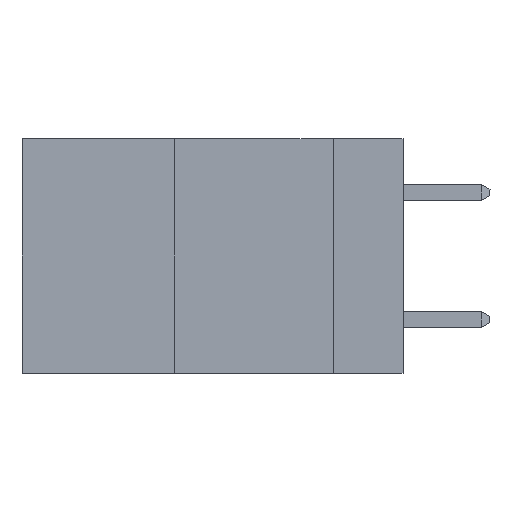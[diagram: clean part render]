
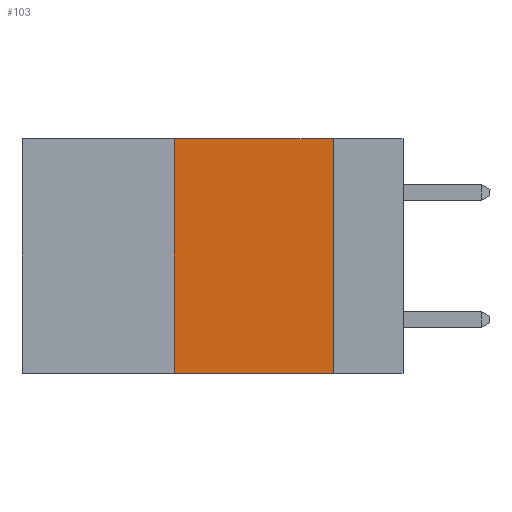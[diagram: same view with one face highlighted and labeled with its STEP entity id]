
A CAD part, left-side view. The second image highlights one B-rep face of the part: STEP entity #103.
In plain terms, the highlighted planar face has unit normal (-1, 0, 0).
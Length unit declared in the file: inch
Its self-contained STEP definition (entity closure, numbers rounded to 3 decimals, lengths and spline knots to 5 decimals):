
#28 = LINE ( 'NONE', #5893, #8463 ) ;
#103 = ADVANCED_FACE ( 'NONE', ( #6063 ), #7456, .F. ) ;
#497 = CARTESIAN_POINT ( 'NONE',  ( 0., 0.36, -0.37 ) ) ;
#874 = CARTESIAN_POINT ( 'NONE',  ( 0., 0.11, 0. ) ) ;
#1186 = VECTOR ( 'NONE', #4324, 39.37008 ) ;
#1333 = VECTOR ( 'NONE', #7448, 39.37008 ) ;
#2434 = LINE ( 'NONE', #874, #10375 ) ;
#2515 = CARTESIAN_POINT ( 'NONE',  ( 0., 0.36, 0. ) ) ;
#3309 = ORIENTED_EDGE ( 'NONE', *, *, #7673, .F. ) ;
#3376 = VERTEX_POINT ( 'NONE', #2515 ) ;
#3705 = LINE ( 'NONE', #4461, #1333 ) ;
#3990 = EDGE_LOOP ( 'NONE', ( #4466, #8824, #3309, #7404 ) ) ;
#4324 = DIRECTION ( 'NONE',  ( 0., 0., 1. ) ) ;
#4461 = CARTESIAN_POINT ( 'NONE',  ( 0., 0.6, -0.37 ) ) ;
#4466 = ORIENTED_EDGE ( 'NONE', *, *, #9819, .F. ) ;
#4814 = AXIS2_PLACEMENT_3D ( 'NONE', #7743, #10152, #10049 ) ;
#4918 = CARTESIAN_POINT ( 'NONE',  ( 0., 0.11, -0.37 ) ) ;
#5893 = CARTESIAN_POINT ( 'NONE',  ( 0., 0.6, 0. ) ) ;
#5933 = DIRECTION ( 'NONE',  ( 0., 0., -1. ) ) ;
#6063 = FACE_OUTER_BOUND ( 'NONE', #3990, .T. ) ;
#6599 = DIRECTION ( 'NONE',  ( 0., -1., 0. ) ) ;
#6814 = VERTEX_POINT ( 'NONE', #4918 ) ;
#7166 = CARTESIAN_POINT ( 'NONE',  ( 0., 0.11, 0. ) ) ;
#7190 = LINE ( 'NONE', #8037, #1186 ) ;
#7404 = ORIENTED_EDGE ( 'NONE', *, *, #7860, .T. ) ;
#7448 = DIRECTION ( 'NONE',  ( 0., -1., 0. ) ) ;
#7456 = PLANE ( 'NONE',  #4814 ) ;
#7673 = EDGE_CURVE ( 'NONE', #10216, #3376, #7190, .T. ) ;
#7743 = CARTESIAN_POINT ( 'NONE',  ( 0., 0.6, 0. ) ) ;
#7748 = EDGE_CURVE ( 'NONE', #3376, #8390, #28, .T. ) ;
#7860 = EDGE_CURVE ( 'NONE', #10216, #6814, #3705, .T. ) ;
#8037 = CARTESIAN_POINT ( 'NONE',  ( 0., 0.36, 0. ) ) ;
#8390 = VERTEX_POINT ( 'NONE', #7166 ) ;
#8463 = VECTOR ( 'NONE', #6599, 39.37008 ) ;
#8824 = ORIENTED_EDGE ( 'NONE', *, *, #7748, .F. ) ;
#9819 = EDGE_CURVE ( 'NONE', #8390, #6814, #2434, .T. ) ;
#10049 = DIRECTION ( 'NONE',  ( 0., 0., -1. ) ) ;
#10152 = DIRECTION ( 'NONE',  ( 1., 0., 0. ) ) ;
#10216 = VERTEX_POINT ( 'NONE', #497 ) ;
#10375 = VECTOR ( 'NONE', #5933, 39.37008 ) ;
